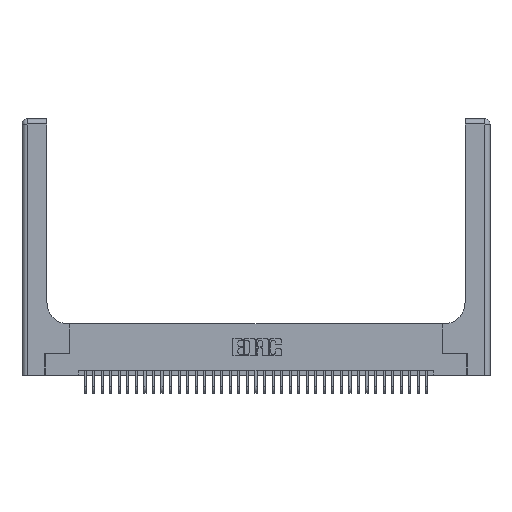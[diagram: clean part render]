
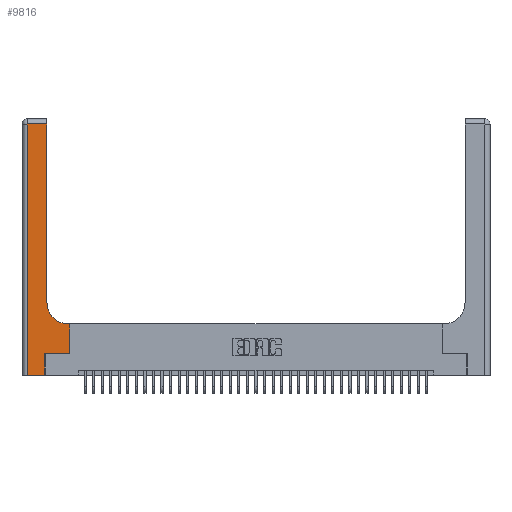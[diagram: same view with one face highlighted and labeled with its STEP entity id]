
A CAD part, top view. The second image highlights one B-rep face of the part: STEP entity #9816.
In plain terms, the highlighted planar face has unit normal (0, 0, 1).
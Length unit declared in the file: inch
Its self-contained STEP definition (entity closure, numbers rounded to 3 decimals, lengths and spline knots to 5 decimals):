
#1034 = ORIENTED_EDGE ( 'NONE', *, *, #36396, .T. ) ;
#1053 = DIRECTION ( 'NONE',  ( 0., 1., 0. ) ) ;
#1403 = EDGE_CURVE ( 'NONE', #34034, #16045, #6741, .T. ) ;
#2211 = VERTEX_POINT ( 'NONE', #30827 ) ;
#2476 = VECTOR ( 'NONE', #6863, 39.37008 ) ;
#3374 = ORIENTED_EDGE ( 'NONE', *, *, #27037, .T. ) ;
#3524 = DIRECTION ( 'NONE',  ( 1., 0., 0. ) ) ;
#3568 = CARTESIAN_POINT ( 'NONE',  ( 0.5415, 0.85, 0.37 ) ) ;
#3691 = AXIS2_PLACEMENT_3D ( 'NONE', #6859, #9927, #31144 ) ;
#3785 = VECTOR ( 'NONE', #34573, 39.37008 ) ;
#4404 = CARTESIAN_POINT ( 'NONE',  ( 0.5585, 0.25, 0.37 ) ) ;
#5272 = ORIENTED_EDGE ( 'NONE', *, *, #1403, .T. ) ;
#5356 = VECTOR ( 'NONE', #37609, 39.37008 ) ;
#6304 = VECTOR ( 'NONE', #19868, 39.37008 ) ;
#6617 = DIRECTION ( 'NONE',  ( 1., 0., 0. ) ) ;
#6741 = LINE ( 'NONE', #15624, #38004 ) ;
#6859 = CARTESIAN_POINT ( 'NONE',  ( 0., 3., 0.37 ) ) ;
#6863 = DIRECTION ( 'NONE',  ( -1., 0., 0. ) ) ;
#6979 = VERTEX_POINT ( 'NONE', #17103 ) ;
#7772 = CARTESIAN_POINT ( 'NONE',  ( 0.2915, 0.6, 0.37 ) ) ;
#7903 = EDGE_LOOP ( 'NONE', ( #16676, #33725, #3374, #5272, #30438, #16214, #1034, #34208, #19041 ) ) ;
#7913 = EDGE_CURVE ( 'NONE', #36484, #15547, #28853, .T. ) ;
#9331 = CARTESIAN_POINT ( 'NONE',  ( 0.06, 2.94, 0.37 ) ) ;
#9801 = CARTESIAN_POINT ( 'NONE',  ( 0., 2.94, 0.37 ) ) ;
#9816 = ADVANCED_FACE ( 'NONE', ( #36161 ), #25019, .F. ) ;
#9927 = DIRECTION ( 'NONE',  ( 0., 0., -1. ) ) ;
#10560 = LINE ( 'NONE', #9801, #2476 ) ;
#10685 = CARTESIAN_POINT ( 'NONE',  ( 0.5585, 0.6, 0.37 ) ) ;
#15013 = LINE ( 'NONE', #31928, #31136 ) ;
#15101 = CARTESIAN_POINT ( 'NONE',  ( 0.2915, 2.94, 0.37 ) ) ;
#15547 = VERTEX_POINT ( 'NONE', #15101 ) ;
#15624 = CARTESIAN_POINT ( 'NONE',  ( 0., 0., 0.37 ) ) ;
#16045 = VERTEX_POINT ( 'NONE', #23259 ) ;
#16161 = CARTESIAN_POINT ( 'NONE',  ( 0.2915, 3., 0.37 ) ) ;
#16214 = ORIENTED_EDGE ( 'NONE', *, *, #31689, .T. ) ;
#16466 = CARTESIAN_POINT ( 'NONE',  ( 0.269, 0.25, 0.37 ) ) ;
#16676 = ORIENTED_EDGE ( 'NONE', *, *, #7913, .T. ) ;
#17103 = CARTESIAN_POINT ( 'NONE',  ( 0.269, 0.25, 0.37 ) ) ;
#17904 = AXIS2_PLACEMENT_3D ( 'NONE', #3568, #24766, #6617 ) ;
#19041 = ORIENTED_EDGE ( 'NONE', *, *, #22196, .T. ) ;
#19868 = DIRECTION ( 'NONE',  ( -1., 0., 0. ) ) ;
#19938 = LINE ( 'NONE', #34455, #3785 ) ;
#20495 = EDGE_CURVE ( 'NONE', #16045, #6979, #15013, .T. ) ;
#22196 = EDGE_CURVE ( 'NONE', #23957, #36484, #27381, .T. ) ;
#23259 = CARTESIAN_POINT ( 'NONE',  ( 0.269, 0., 0.37 ) ) ;
#23957 = VERTEX_POINT ( 'NONE', #35157 ) ;
#24766 = DIRECTION ( 'NONE',  ( 0., 0., -1. ) ) ;
#25019 = PLANE ( 'NONE',  #3691 ) ;
#25295 = EDGE_CURVE ( 'NONE', #35882, #23957, #38493, .T. ) ;
#26030 = CARTESIAN_POINT ( 'NONE',  ( 0.2915, 0.85, 0.37 ) ) ;
#26716 = LINE ( 'NONE', #4404, #33806 ) ;
#27037 = EDGE_CURVE ( 'NONE', #34397, #34034, #19938, .T. ) ;
#27381 = CIRCLE ( 'NONE', #17904, 0.25 ) ;
#27676 = LINE ( 'NONE', #16466, #5356 ) ;
#27905 = VECTOR ( 'NONE', #1053, 39.37008 ) ;
#28853 = LINE ( 'NONE', #16161, #27905 ) ;
#30438 = ORIENTED_EDGE ( 'NONE', *, *, #20495, .T. ) ;
#30827 = CARTESIAN_POINT ( 'NONE',  ( 0.5585, 0.25, 0.37 ) ) ;
#31007 = CARTESIAN_POINT ( 'NONE',  ( 0.06, 0., 0.37 ) ) ;
#31136 = VECTOR ( 'NONE', #34963, 39.37008 ) ;
#31144 = DIRECTION ( 'NONE',  ( -1., 0., 0. ) ) ;
#31689 = EDGE_CURVE ( 'NONE', #6979, #2211, #27676, .T. ) ;
#31928 = CARTESIAN_POINT ( 'NONE',  ( 0.269, 0., 0.37 ) ) ;
#32144 = EDGE_CURVE ( 'NONE', #15547, #34397, #10560, .T. ) ;
#33725 = ORIENTED_EDGE ( 'NONE', *, *, #32144, .T. ) ;
#33806 = VECTOR ( 'NONE', #37507, 39.37008 ) ;
#34034 = VERTEX_POINT ( 'NONE', #31007 ) ;
#34208 = ORIENTED_EDGE ( 'NONE', *, *, #25295, .T. ) ;
#34397 = VERTEX_POINT ( 'NONE', #9331 ) ;
#34455 = CARTESIAN_POINT ( 'NONE',  ( 0.06, 3., 0.37 ) ) ;
#34573 = DIRECTION ( 'NONE',  ( 0., -1., 0. ) ) ;
#34963 = DIRECTION ( 'NONE',  ( 0., 1., 0. ) ) ;
#35157 = CARTESIAN_POINT ( 'NONE',  ( 0.5415, 0.6, 0.37 ) ) ;
#35882 = VERTEX_POINT ( 'NONE', #10685 ) ;
#36161 = FACE_OUTER_BOUND ( 'NONE', #7903, .T. ) ;
#36396 = EDGE_CURVE ( 'NONE', #2211, #35882, #26716, .T. ) ;
#36484 = VERTEX_POINT ( 'NONE', #26030 ) ;
#37507 = DIRECTION ( 'NONE',  ( 0., 1., 0. ) ) ;
#37609 = DIRECTION ( 'NONE',  ( 1., 0., 0. ) ) ;
#38004 = VECTOR ( 'NONE', #3524, 39.37008 ) ;
#38493 = LINE ( 'NONE', #7772, #6304 ) ;
